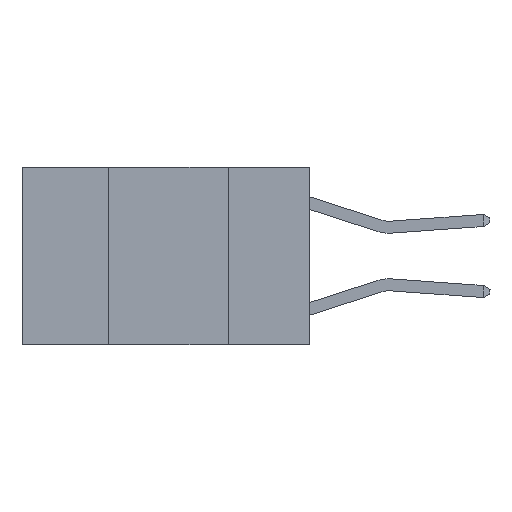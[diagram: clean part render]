
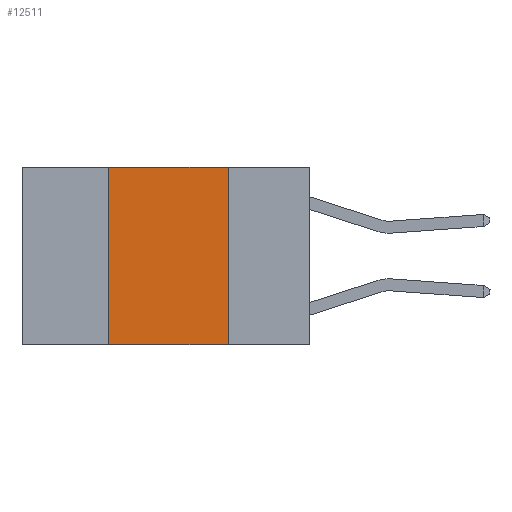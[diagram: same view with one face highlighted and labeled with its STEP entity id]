
A CAD part, left-side view. The second image highlights one B-rep face of the part: STEP entity #12511.
In plain terms, the highlighted planar face has unit normal (-1, 0, 0).
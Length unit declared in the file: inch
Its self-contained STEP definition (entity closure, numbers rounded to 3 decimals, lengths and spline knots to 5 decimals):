
#15 = EDGE_CURVE ( 'NONE', #16871, #25848, #8005, .T. ) ;
#113 = VECTOR ( 'NONE', #19103, 39.37008 ) ;
#978 = CARTESIAN_POINT ( 'NONE',  ( 0., 0.42, -0.37 ) ) ;
#2508 = ORIENTED_EDGE ( 'NONE', *, *, #16172, .F. ) ;
#4642 = EDGE_CURVE ( 'NONE', #17566, #17921, #22731, .T. ) ;
#5607 = LINE ( 'NONE', #17025, #113 ) ;
#6115 = DIRECTION ( 'NONE',  ( 0., -1., 0. ) ) ;
#6159 = CARTESIAN_POINT ( 'NONE',  ( 0., 0.17, 0. ) ) ;
#6889 = VECTOR ( 'NONE', #6115, 39.37008 ) ;
#7159 = CARTESIAN_POINT ( 'NONE',  ( 0., 0.42, 0. ) ) ;
#8005 = LINE ( 'NONE', #18548, #12849 ) ;
#9052 = CARTESIAN_POINT ( 'NONE',  ( 0., 0.17, -0.37 ) ) ;
#9258 = FACE_OUTER_BOUND ( 'NONE', #23009, .T. ) ;
#9622 = ORIENTED_EDGE ( 'NONE', *, *, #14251, .F. ) ;
#9729 = CARTESIAN_POINT ( 'NONE',  ( 0., 0.6, 0. ) ) ;
#11813 = DIRECTION ( 'NONE',  ( 1., 0., 0. ) ) ;
#12511 = ADVANCED_FACE ( 'NONE', ( #9258 ), #22071, .F. ) ;
#12849 = VECTOR ( 'NONE', #14408, 39.37008 ) ;
#13205 = CARTESIAN_POINT ( 'NONE',  ( 0., 0.42, 0. ) ) ;
#14251 = EDGE_CURVE ( 'NONE', #17921, #25848, #5607, .T. ) ;
#14408 = DIRECTION ( 'NONE',  ( 0., -1., 0. ) ) ;
#14607 = AXIS2_PLACEMENT_3D ( 'NONE', #9729, #11813, #26282 ) ;
#16172 = EDGE_CURVE ( 'NONE', #16871, #17566, #23590, .T. ) ;
#16871 = VERTEX_POINT ( 'NONE', #978 ) ;
#17025 = CARTESIAN_POINT ( 'NONE',  ( 0., 0.17, 0. ) ) ;
#17566 = VERTEX_POINT ( 'NONE', #7159 ) ;
#17921 = VERTEX_POINT ( 'NONE', #6159 ) ;
#18347 = ORIENTED_EDGE ( 'NONE', *, *, #4642, .F. ) ;
#18548 = CARTESIAN_POINT ( 'NONE',  ( 0., 0.6, -0.37 ) ) ;
#19103 = DIRECTION ( 'NONE',  ( 0., 0., -1. ) ) ;
#19622 = ORIENTED_EDGE ( 'NONE', *, *, #15, .T. ) ;
#20554 = CARTESIAN_POINT ( 'NONE',  ( 0., 0.6, 0. ) ) ;
#21478 = DIRECTION ( 'NONE',  ( 0., 0., 1. ) ) ;
#22071 = PLANE ( 'NONE',  #14607 ) ;
#22731 = LINE ( 'NONE', #20554, #6889 ) ;
#22932 = VECTOR ( 'NONE', #21478, 39.37008 ) ;
#23009 = EDGE_LOOP ( 'NONE', ( #9622, #18347, #2508, #19622 ) ) ;
#23590 = LINE ( 'NONE', #13205, #22932 ) ;
#25848 = VERTEX_POINT ( 'NONE', #9052 ) ;
#26282 = DIRECTION ( 'NONE',  ( 0., 0., -1. ) ) ;
